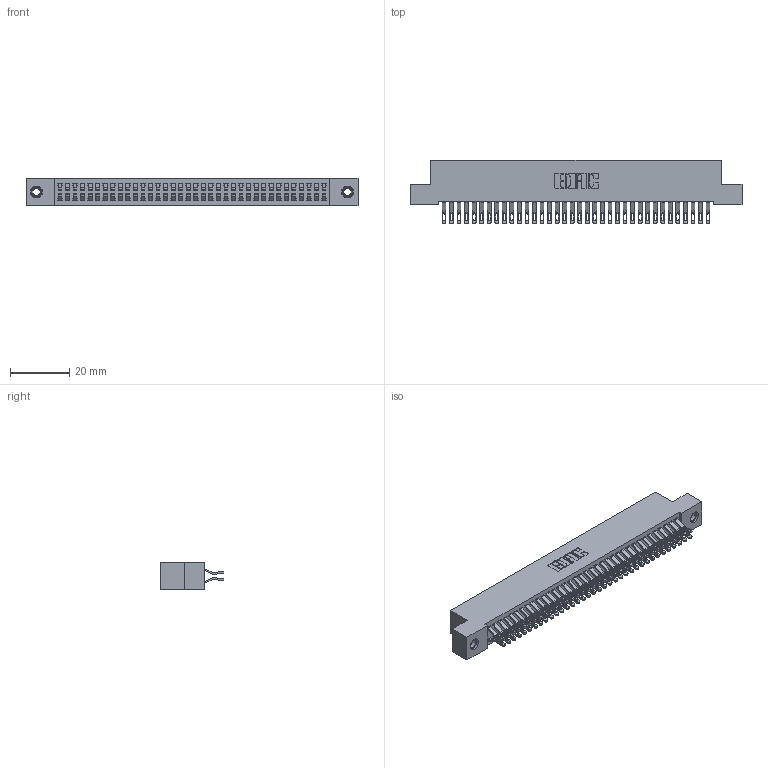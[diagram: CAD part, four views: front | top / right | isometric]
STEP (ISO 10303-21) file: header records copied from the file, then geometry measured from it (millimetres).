
FILE_DESCRIPTION (( 'STEP AP203' ), '1' );
FILE_NAME ('392-072-555-207.STEP', '2019-10-09T12:40:01', ( '' ), ( '' ), 'SwSTEP 2.0', 'SolidWorks 2016', '' );
FILE_SCHEMA (( 'CONFIG_CONTROL_DESIGN' ));
Length unit declared in the file: inch
Products named in the file (4): 392-072-555-207; 342 Part_TI; 345-292-001_555 Tail; 345-250-001_345-250-005-103
Assembly tree (75 placements, depth 2):
  392-072-555-207
    342 Part_TI
    345-292-001_555 Tail  x72
    345-250-001_345-250-005-103  x2
Bounding box: 111.76 x 21.47 x 9.4 mm (x, y, z)
Volume: 10200.6 mm3; surface area: 17178.6 mm2
Topology: 75 solids, 75 shells, 4346 faces, 13611 edges, 9066 vertices
Faces by surface type: plane 2546, cylinder 1784, cone 12, torus 4
Entity records: 25316 total; most frequent: CARTESIAN_POINT 4219, ORIENTED_EDGE 4118, DIRECTION 3617, EDGE_CURVE 2059, VECTOR 1891, LINE 1891, VERTEX_POINT 1368, AXIS2_PLACEMENT_3D 863
